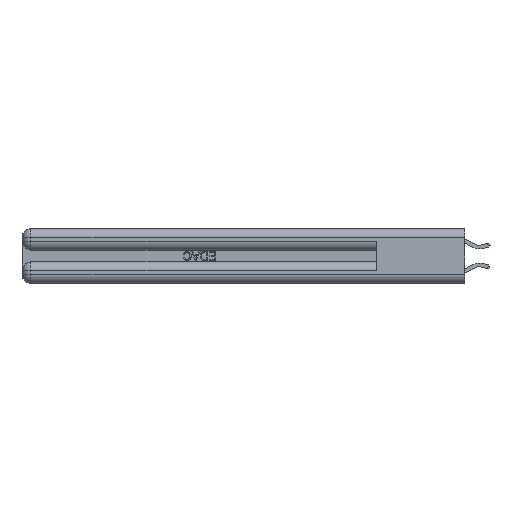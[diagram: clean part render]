
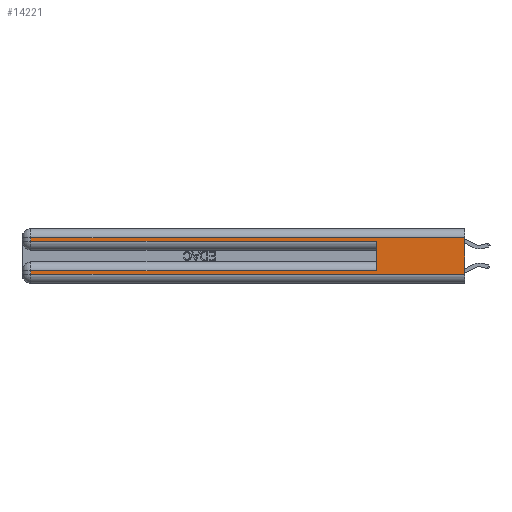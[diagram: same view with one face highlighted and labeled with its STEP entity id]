
A CAD part, left-side view. The second image highlights one B-rep face of the part: STEP entity #14221.
In plain terms, the highlighted planar face has unit normal (-1, 0, 0).
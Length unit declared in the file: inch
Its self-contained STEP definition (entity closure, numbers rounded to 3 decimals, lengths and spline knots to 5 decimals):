
#115 = LINE ( 'NONE', #14245, #17089 ) ;
#222 = VERTEX_POINT ( 'NONE', #21432 ) ;
#227 = DIRECTION ( 'NONE',  ( 0., 0., -1. ) ) ;
#736 = CARTESIAN_POINT ( 'NONE',  ( 0., 2.94, 0.31 ) ) ;
#1264 = DIRECTION ( 'NONE',  ( 1., 0., 0. ) ) ;
#1804 = ORIENTED_EDGE ( 'NONE', *, *, #15762, .F. ) ;
#2534 = CARTESIAN_POINT ( 'NONE',  ( 0., 2.94, 0.37 ) ) ;
#3712 = VECTOR ( 'NONE', #26612, 39.37008 ) ;
#4473 = CARTESIAN_POINT ( 'NONE',  ( 0., 0., 0.31 ) ) ;
#4938 = ORIENTED_EDGE ( 'NONE', *, *, #11648, .T. ) ;
#4942 = AXIS2_PLACEMENT_3D ( 'NONE', #28885, #1264, #31641 ) ;
#5241 = VERTEX_POINT ( 'NONE', #31110 ) ;
#5558 = VECTOR ( 'NONE', #227, 39.37008 ) ;
#6405 = VECTOR ( 'NONE', #16414, 39.37008 ) ;
#8770 = CARTESIAN_POINT ( 'NONE',  ( 0., 2.94, 0.37 ) ) ;
#9646 = CARTESIAN_POINT ( 'NONE',  ( 0., 0., 0.31 ) ) ;
#10000 = FACE_OUTER_BOUND ( 'NONE', #30276, .T. ) ;
#10221 = EDGE_CURVE ( 'NONE', #11256, #14354, #115, .T. ) ;
#10428 = DIRECTION ( 'NONE',  ( 0., 0., 1. ) ) ;
#10459 = DIRECTION ( 'NONE',  ( 0., -1., 0. ) ) ;
#11035 = ORIENTED_EDGE ( 'NONE', *, *, #26614, .F. ) ;
#11256 = VERTEX_POINT ( 'NONE', #18881 ) ;
#11648 = EDGE_CURVE ( 'NONE', #17220, #222, #23517, .T. ) ;
#11951 = VECTOR ( 'NONE', #10459, 39.37008 ) ;
#12148 = ORIENTED_EDGE ( 'NONE', *, *, #23429, .T. ) ;
#12784 = VERTEX_POINT ( 'NONE', #18519 ) ;
#13826 = LINE ( 'NONE', #35406, #19459 ) ;
#14221 = ADVANCED_FACE ( 'NONE', ( #10000 ), #26102, .F. ) ;
#14245 = CARTESIAN_POINT ( 'NONE',  ( 0., 0., 0.06 ) ) ;
#14354 = VERTEX_POINT ( 'NONE', #23577 ) ;
#14845 = ORIENTED_EDGE ( 'NONE', *, *, #16696, .T. ) ;
#15536 = DIRECTION ( 'NONE',  ( 0., 0., -1. ) ) ;
#15762 = EDGE_CURVE ( 'NONE', #18414, #14354, #22485, .T. ) ;
#15800 = ORIENTED_EDGE ( 'NONE', *, *, #10221, .T. ) ;
#16289 = CARTESIAN_POINT ( 'NONE',  ( 0., 0., 0.085 ) ) ;
#16396 = DIRECTION ( 'NONE',  ( 0., 0., -1. ) ) ;
#16414 = DIRECTION ( 'NONE',  ( 0., 1., 0. ) ) ;
#16696 = EDGE_CURVE ( 'NONE', #18414, #17220, #29809, .T. ) ;
#17089 = VECTOR ( 'NONE', #30894, 39.37008 ) ;
#17220 = VERTEX_POINT ( 'NONE', #736 ) ;
#18414 = VERTEX_POINT ( 'NONE', #9646 ) ;
#18519 = CARTESIAN_POINT ( 'NONE',  ( 0., 0.6, 0.285 ) ) ;
#18881 = CARTESIAN_POINT ( 'NONE',  ( 0., 2.94, 0.06 ) ) ;
#19459 = VECTOR ( 'NONE', #10428, 39.37008 ) ;
#21432 = CARTESIAN_POINT ( 'NONE',  ( 0., 2.94, 0.285 ) ) ;
#22485 = LINE ( 'NONE', #32142, #24257 ) ;
#23429 = EDGE_CURVE ( 'NONE', #5241, #11256, #33359, .T. ) ;
#23517 = LINE ( 'NONE', #2534, #27449 ) ;
#23577 = CARTESIAN_POINT ( 'NONE',  ( 0., 0., 0.06 ) ) ;
#23669 = EDGE_CURVE ( 'NONE', #26434, #5241, #29859, .T. ) ;
#24257 = VECTOR ( 'NONE', #15536, 39.37008 ) ;
#26102 = PLANE ( 'NONE',  #4942 ) ;
#26434 = VERTEX_POINT ( 'NONE', #31461 ) ;
#26612 = DIRECTION ( 'NONE',  ( 0., 1., 0. ) ) ;
#26614 = EDGE_CURVE ( 'NONE', #26434, #12784, #13826, .T. ) ;
#26666 = CARTESIAN_POINT ( 'NONE',  ( 0., 0., 0.285 ) ) ;
#27449 = VECTOR ( 'NONE', #16396, 39.37008 ) ;
#27951 = EDGE_CURVE ( 'NONE', #222, #12784, #34552, .T. ) ;
#28885 = CARTESIAN_POINT ( 'NONE',  ( 0., 0., 0.37 ) ) ;
#29809 = LINE ( 'NONE', #4473, #3712 ) ;
#29859 = LINE ( 'NONE', #16289, #6405 ) ;
#30276 = EDGE_LOOP ( 'NONE', ( #1804, #14845, #4938, #30315, #11035, #34854, #12148, #15800 ) ) ;
#30315 = ORIENTED_EDGE ( 'NONE', *, *, #27951, .T. ) ;
#30894 = DIRECTION ( 'NONE',  ( 0., -1., 0. ) ) ;
#31110 = CARTESIAN_POINT ( 'NONE',  ( 0., 2.94, 0.085 ) ) ;
#31461 = CARTESIAN_POINT ( 'NONE',  ( 0., 0.6, 0.085 ) ) ;
#31641 = DIRECTION ( 'NONE',  ( 0., 0., -1. ) ) ;
#32142 = CARTESIAN_POINT ( 'NONE',  ( 0., 0., 0.37 ) ) ;
#33359 = LINE ( 'NONE', #8770, #5558 ) ;
#34552 = LINE ( 'NONE', #26666, #11951 ) ;
#34854 = ORIENTED_EDGE ( 'NONE', *, *, #23669, .T. ) ;
#35406 = CARTESIAN_POINT ( 'NONE',  ( 0., 0.6, 0.145 ) ) ;
